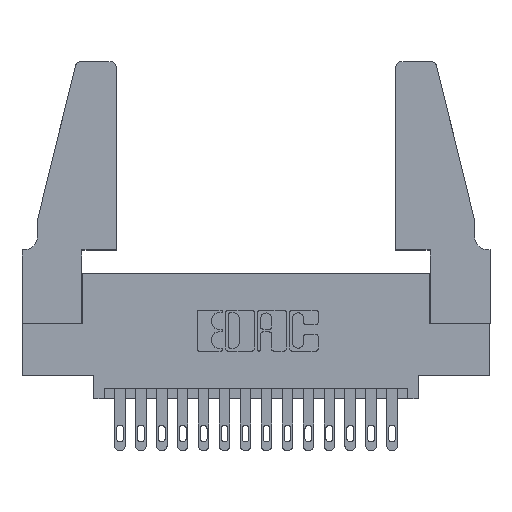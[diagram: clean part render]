
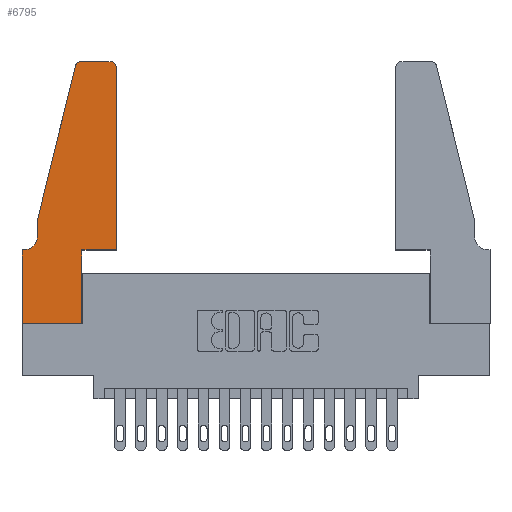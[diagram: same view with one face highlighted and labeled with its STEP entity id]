
A CAD part, top view. The second image highlights one B-rep face of the part: STEP entity #6795.
In plain terms, the highlighted planar face has unit normal (0, 0, 1).
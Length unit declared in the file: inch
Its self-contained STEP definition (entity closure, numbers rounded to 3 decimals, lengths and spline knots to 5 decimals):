
#143 = VERTEX_POINT ( 'NONE', #12120 ) ;
#208 = DIRECTION ( 'NONE',  ( 0., 0., 1. ) ) ;
#461 = CARTESIAN_POINT ( 'NONE',  ( 0.2865, 0.35, 0.37 ) ) ;
#772 = DIRECTION ( 'NONE',  ( 0., 0., 1. ) ) ;
#972 = CIRCLE ( 'NONE', #11839, 0.03 ) ;
#999 = CARTESIAN_POINT ( 'NONE',  ( 0.2865, 0., 0.37 ) ) ;
#1015 = CARTESIAN_POINT ( 'NONE',  ( 0.2865, 0.35, 0.37 ) ) ;
#1253 = DIRECTION ( 'NONE',  ( 1., 0., 0. ) ) ;
#1338 = CARTESIAN_POINT ( 'NONE',  ( 0.284, 1.22, 0.37 ) ) ;
#1393 = CARTESIAN_POINT ( 'NONE',  ( 0.284, 1.25, 0.37 ) ) ;
#1779 = LINE ( 'NONE', #11475, #9766 ) ;
#1780 = DIRECTION ( 'NONE',  ( 0., 1., 0. ) ) ;
#1862 = EDGE_CURVE ( 'NONE', #143, #8797, #9418, .T. ) ;
#2075 = VERTEX_POINT ( 'NONE', #999 ) ;
#2147 = LINE ( 'NONE', #13154, #12780 ) ;
#2415 = DIRECTION ( 'NONE',  ( -1., 0., 0. ) ) ;
#2499 = VERTEX_POINT ( 'NONE', #14151 ) ;
#2676 = DIRECTION ( 'NONE',  ( 1., 0., 0. ) ) ;
#2724 = VERTEX_POINT ( 'NONE', #12982 ) ;
#3000 = EDGE_CURVE ( 'NONE', #2075, #16105, #5657, .T. ) ;
#3292 = VECTOR ( 'NONE', #7605, 39.37008 ) ;
#3492 = DIRECTION ( 'NONE',  ( -1., 0., 0. ) ) ;
#3894 = ORIENTED_EDGE ( 'NONE', *, *, #7314, .T. ) ;
#3984 = DIRECTION ( 'NONE',  ( 1., 0., 0. ) ) ;
#4260 = VECTOR ( 'NONE', #5133, 39.37008 ) ;
#4615 = AXIS2_PLACEMENT_3D ( 'NONE', #1338, #14467, #2676 ) ;
#4702 = CARTESIAN_POINT ( 'NONE',  ( 0.25487, 1.22718, 0.37 ) ) ;
#4790 = EDGE_CURVE ( 'NONE', #8797, #8512, #972, .T. ) ;
#5133 = DIRECTION ( 'NONE',  ( 0., 1., 0. ) ) ;
#5249 = CARTESIAN_POINT ( 'NONE',  ( 0.4505, 1.22, 0.37 ) ) ;
#5289 = CIRCLE ( 'NONE', #4615, 0.03 ) ;
#5657 = LINE ( 'NONE', #461, #10002 ) ;
#5736 = LINE ( 'NONE', #5952, #12121 ) ;
#5952 = CARTESIAN_POINT ( 'NONE',  ( 0.0755, 0.5, 0.37 ) ) ;
#6021 = ORIENTED_EDGE ( 'NONE', *, *, #14098, .T. ) ;
#6285 = EDGE_CURVE ( 'NONE', #14856, #2075, #2147, .T. ) ;
#6303 = CARTESIAN_POINT ( 'NONE',  ( 0., 0., 0.37 ) ) ;
#6630 = ORIENTED_EDGE ( 'NONE', *, *, #12131, .T. ) ;
#6795 = ADVANCED_FACE ( 'NONE', ( #12763 ), #16159, .T. ) ;
#6911 = EDGE_CURVE ( 'NONE', #8512, #12111, #11114, .T. ) ;
#7174 = VECTOR ( 'NONE', #16852, 39.37008 ) ;
#7314 = EDGE_CURVE ( 'NONE', #10886, #10134, #11925, .T. ) ;
#7460 = CARTESIAN_POINT ( 'NONE',  ( 0.0755, 0.35, 0.37 ) ) ;
#7507 = LINE ( 'NONE', #7460, #13271 ) ;
#7579 = ORIENTED_EDGE ( 'NONE', *, *, #6911, .T. ) ;
#7605 = DIRECTION ( 'NONE',  ( -0.239, -0.971, 0. ) ) ;
#7925 = CARTESIAN_POINT ( 'NONE',  ( 0.4505, 0.35, 0.37 ) ) ;
#7967 = DIRECTION ( 'NONE',  ( -1., 0., 0. ) ) ;
#8268 = CARTESIAN_POINT ( 'NONE',  ( 0., 0.35, 0.37 ) ) ;
#8408 = AXIS2_PLACEMENT_3D ( 'NONE', #8879, #13012, #2415 ) ;
#8512 = VERTEX_POINT ( 'NONE', #16129 ) ;
#8605 = DIRECTION ( 'NONE',  ( 0., -1., 0. ) ) ;
#8797 = VERTEX_POINT ( 'NONE', #5249 ) ;
#8879 = CARTESIAN_POINT ( 'NONE',  ( 0.0055, 0.42, 0.37 ) ) ;
#8919 = ORIENTED_EDGE ( 'NONE', *, *, #6285, .T. ) ;
#9301 = CARTESIAN_POINT ( 'NONE',  ( 0.0755, 0.5, 0.37 ) ) ;
#9418 = LINE ( 'NONE', #7925, #4260 ) ;
#9604 = DIRECTION ( 'NONE',  ( 1., 0., 0. ) ) ;
#9766 = VECTOR ( 'NONE', #1253, 39.37008 ) ;
#9831 = ORIENTED_EDGE ( 'NONE', *, *, #11227, .T. ) ;
#9954 = AXIS2_PLACEMENT_3D ( 'NONE', #8268, #772, #9604 ) ;
#10002 = VECTOR ( 'NONE', #1780, 39.37008 ) ;
#10127 = ORIENTED_EDGE ( 'NONE', *, *, #16067, .T. ) ;
#10134 = VERTEX_POINT ( 'NONE', #9301 ) ;
#10813 = ORIENTED_EDGE ( 'NONE', *, *, #3000, .T. ) ;
#10886 = VERTEX_POINT ( 'NONE', #4702 ) ;
#11114 = LINE ( 'NONE', #15742, #15472 ) ;
#11227 = EDGE_CURVE ( 'NONE', #10134, #2499, #5736, .T. ) ;
#11475 = CARTESIAN_POINT ( 'NONE',  ( 0.4505, 0.35, 0.37 ) ) ;
#11804 = CARTESIAN_POINT ( 'NONE',  ( 0.4205, 1.22, 0.37 ) ) ;
#11839 = AXIS2_PLACEMENT_3D ( 'NONE', #11804, #208, #3984 ) ;
#11925 = LINE ( 'NONE', #12592, #3292 ) ;
#12077 = EDGE_LOOP ( 'NONE', ( #7579, #6630, #3894, #9831, #10127, #14570, #16189, #8919, #10813, #6021, #13196, #12093 ) ) ;
#12087 = LINE ( 'NONE', #6303, #7174 ) ;
#12093 = ORIENTED_EDGE ( 'NONE', *, *, #4790, .T. ) ;
#12111 = VERTEX_POINT ( 'NONE', #1393 ) ;
#12120 = CARTESIAN_POINT ( 'NONE',  ( 0.4505, 0.35, 0.37 ) ) ;
#12121 = VECTOR ( 'NONE', #8605, 39.37008 ) ;
#12131 = EDGE_CURVE ( 'NONE', #12111, #10886, #5289, .T. ) ;
#12267 = DIRECTION ( 'NONE',  ( 1., 0., 0. ) ) ;
#12592 = CARTESIAN_POINT ( 'NONE',  ( 0.0755, 0.5, 0.37 ) ) ;
#12763 = FACE_OUTER_BOUND ( 'NONE', #12077, .T. ) ;
#12780 = VECTOR ( 'NONE', #12267, 39.37008 ) ;
#12982 = CARTESIAN_POINT ( 'NONE',  ( 0., 0.35, 0.37 ) ) ;
#13012 = DIRECTION ( 'NONE',  ( 0., 0., -1. ) ) ;
#13154 = CARTESIAN_POINT ( 'NONE',  ( 0., 0., 0.37 ) ) ;
#13196 = ORIENTED_EDGE ( 'NONE', *, *, #1862, .T. ) ;
#13271 = VECTOR ( 'NONE', #3492, 39.37008 ) ;
#13928 = CARTESIAN_POINT ( 'NONE',  ( 0., 0., 0.37 ) ) ;
#14048 = EDGE_CURVE ( 'NONE', #16923, #2724, #7507, .T. ) ;
#14098 = EDGE_CURVE ( 'NONE', #16105, #143, #1779, .T. ) ;
#14151 = CARTESIAN_POINT ( 'NONE',  ( 0.0755, 0.42, 0.37 ) ) ;
#14467 = DIRECTION ( 'NONE',  ( 0., 0., 1. ) ) ;
#14570 = ORIENTED_EDGE ( 'NONE', *, *, #14048, .T. ) ;
#14856 = VERTEX_POINT ( 'NONE', #13928 ) ;
#15472 = VECTOR ( 'NONE', #7967, 39.37008 ) ;
#15742 = CARTESIAN_POINT ( 'NONE',  ( 0.2605, 1.25, 0.37 ) ) ;
#16024 = EDGE_CURVE ( 'NONE', #2724, #14856, #12087, .T. ) ;
#16037 = CIRCLE ( 'NONE', #8408, 0.07 ) ;
#16067 = EDGE_CURVE ( 'NONE', #2499, #16923, #16037, .T. ) ;
#16105 = VERTEX_POINT ( 'NONE', #1015 ) ;
#16129 = CARTESIAN_POINT ( 'NONE',  ( 0.4205, 1.25, 0.37 ) ) ;
#16159 = PLANE ( 'NONE',  #9954 ) ;
#16189 = ORIENTED_EDGE ( 'NONE', *, *, #16024, .T. ) ;
#16650 = CARTESIAN_POINT ( 'NONE',  ( 0.0055, 0.35, 0.37 ) ) ;
#16852 = DIRECTION ( 'NONE',  ( 0., -1., 0. ) ) ;
#16923 = VERTEX_POINT ( 'NONE', #16650 ) ;
